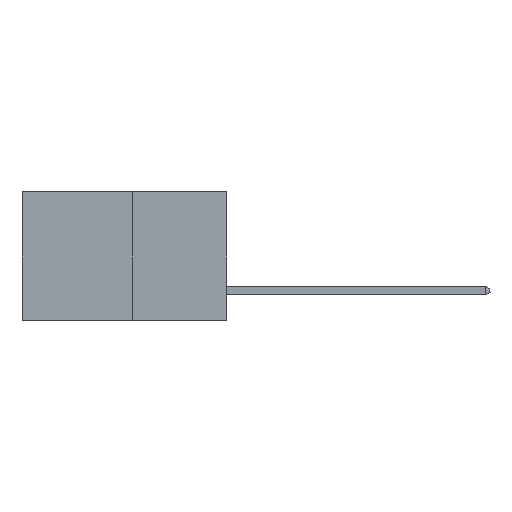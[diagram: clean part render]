
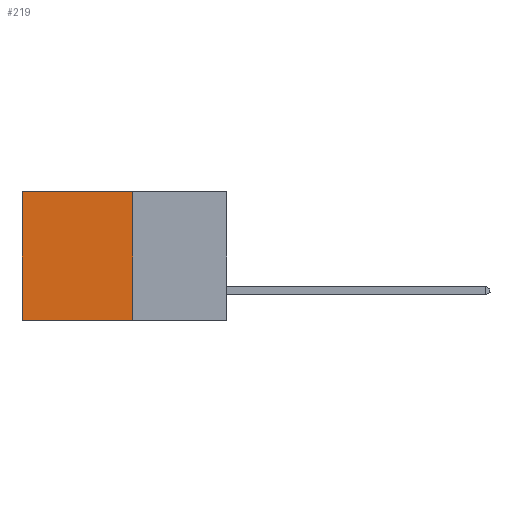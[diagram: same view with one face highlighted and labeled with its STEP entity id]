
A CAD part, left-side view. The second image highlights one B-rep face of the part: STEP entity #219.
In plain terms, the highlighted planar face has unit normal (-1, 0, 0).
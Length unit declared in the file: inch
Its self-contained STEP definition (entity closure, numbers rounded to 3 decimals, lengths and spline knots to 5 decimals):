
#90 = ORIENTED_EDGE ( 'NONE', *, *, #3082, .T. ) ;
#137 = CARTESIAN_POINT ( 'NONE',  ( 0.277, 0.59, -0.37 ) ) ;
#190 = VERTEX_POINT ( 'NONE', #8381 ) ;
#219 = ADVANCED_FACE ( 'NONE', ( #1051 ), #694, .F. ) ;
#308 = EDGE_LOOP ( 'NONE', ( #90, #8031, #4566, #6899 ) ) ;
#538 = VERTEX_POINT ( 'NONE', #137 ) ;
#634 = CARTESIAN_POINT ( 'NONE',  ( 0.277, 0.27, -0.37 ) ) ;
#651 = CARTESIAN_POINT ( 'NONE',  ( 0.277, 0.27, -0.37 ) ) ;
#694 = PLANE ( 'NONE',  #4277 ) ;
#1051 = FACE_OUTER_BOUND ( 'NONE', #308, .T. ) ;
#1052 = LINE ( 'NONE', #651, #2632 ) ;
#1827 = EDGE_CURVE ( 'NONE', #3893, #190, #7890, .T. ) ;
#1845 = DIRECTION ( 'NONE',  ( 1., 0., 0. ) ) ;
#1932 = CARTESIAN_POINT ( 'NONE',  ( 0.277, 0.27, 0. ) ) ;
#1940 = DIRECTION ( 'NONE',  ( 0., 1., 0. ) ) ;
#2330 = CARTESIAN_POINT ( 'NONE',  ( 0.277, 0.27, 0. ) ) ;
#2372 = DIRECTION ( 'NONE',  ( 0., 1., 0. ) ) ;
#2632 = VECTOR ( 'NONE', #1940, 39.37008 ) ;
#2900 = VECTOR ( 'NONE', #4815, 39.37008 ) ;
#2907 = VERTEX_POINT ( 'NONE', #4780 ) ;
#3082 = EDGE_CURVE ( 'NONE', #190, #538, #8054, .T. ) ;
#3129 = EDGE_CURVE ( 'NONE', #3893, #2907, #7314, .T. ) ;
#3893 = VERTEX_POINT ( 'NONE', #1932 ) ;
#3933 = VECTOR ( 'NONE', #5177, 39.37008 ) ;
#3956 = DIRECTION ( 'NONE',  ( 0., 0., -1. ) ) ;
#4277 = AXIS2_PLACEMENT_3D ( 'NONE', #634, #1845, #3956 ) ;
#4379 = EDGE_CURVE ( 'NONE', #2907, #538, #1052, .T. ) ;
#4566 = ORIENTED_EDGE ( 'NONE', *, *, #3129, .F. ) ;
#4641 = VECTOR ( 'NONE', #2372, 39.37008 ) ;
#4780 = CARTESIAN_POINT ( 'NONE',  ( 0.277, 0.27, -0.37 ) ) ;
#4815 = DIRECTION ( 'NONE',  ( 0., 0., -1. ) ) ;
#4850 = CARTESIAN_POINT ( 'NONE',  ( 0.277, 0.59, -0.37 ) ) ;
#5177 = DIRECTION ( 'NONE',  ( 0., 0., -1. ) ) ;
#5426 = CARTESIAN_POINT ( 'NONE',  ( 0.277, 0.27, -0.37 ) ) ;
#6899 = ORIENTED_EDGE ( 'NONE', *, *, #1827, .T. ) ;
#7314 = LINE ( 'NONE', #5426, #3933 ) ;
#7890 = LINE ( 'NONE', #2330, #4641 ) ;
#8031 = ORIENTED_EDGE ( 'NONE', *, *, #4379, .F. ) ;
#8054 = LINE ( 'NONE', #4850, #2900 ) ;
#8381 = CARTESIAN_POINT ( 'NONE',  ( 0.277, 0.59, 0. ) ) ;
